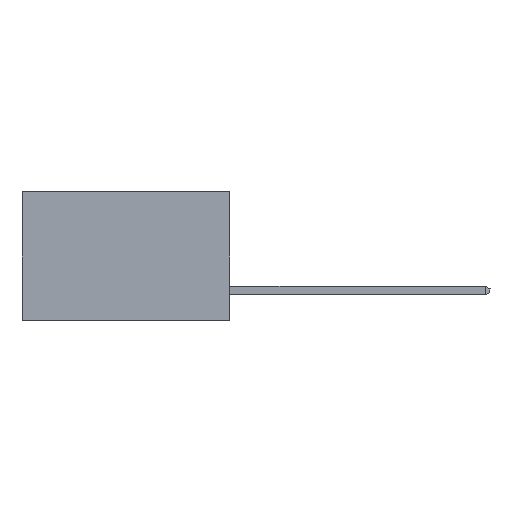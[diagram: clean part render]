
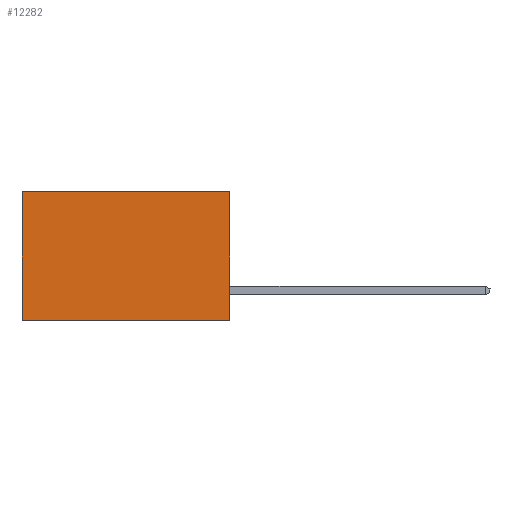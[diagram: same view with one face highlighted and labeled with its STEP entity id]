
A CAD part, left-side view. The second image highlights one B-rep face of the part: STEP entity #12282.
In plain terms, the highlighted planar face has unit normal (-1, 0, 0).
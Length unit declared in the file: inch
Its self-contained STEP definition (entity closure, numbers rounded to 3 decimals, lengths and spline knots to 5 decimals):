
#436 = LINE ( 'NONE', #7657, #5934 ) ;
#659 = ORIENTED_EDGE ( 'NONE', *, *, #10849, .F. ) ;
#1196 = LINE ( 'NONE', #14230, #4941 ) ;
#1981 = ORIENTED_EDGE ( 'NONE', *, *, #10975, .F. ) ;
#3403 = CARTESIAN_POINT ( 'NONE',  ( 0.2615, 0., -0.37 ) ) ;
#3485 = CARTESIAN_POINT ( 'NONE',  ( 0.2615, 0., -0.37 ) ) ;
#4744 = VERTEX_POINT ( 'NONE', #11802 ) ;
#4941 = VECTOR ( 'NONE', #8578, 39.37008 ) ;
#5934 = VECTOR ( 'NONE', #12455, 39.37008 ) ;
#6641 = EDGE_LOOP ( 'NONE', ( #12368, #1981, #659, #8754 ) ) ;
#7217 = EDGE_CURVE ( 'NONE', #10637, #8320, #1196, .T. ) ;
#7335 = CARTESIAN_POINT ( 'NONE',  ( 0.2615, 0.6, 0. ) ) ;
#7657 = CARTESIAN_POINT ( 'NONE',  ( 0.2615, 0., -0.37 ) ) ;
#8320 = VERTEX_POINT ( 'NONE', #14591 ) ;
#8326 = DIRECTION ( 'NONE',  ( 1., 0., 0. ) ) ;
#8578 = DIRECTION ( 'NONE',  ( 0., 0., -1. ) ) ;
#8694 = AXIS2_PLACEMENT_3D ( 'NONE', #3485, #8326, #13577 ) ;
#8754 = ORIENTED_EDGE ( 'NONE', *, *, #12151, .T. ) ;
#9497 = FACE_OUTER_BOUND ( 'NONE', #6641, .T. ) ;
#9571 = DIRECTION ( 'NONE',  ( 0., 0., -1. ) ) ;
#9938 = VECTOR ( 'NONE', #9571, 39.37008 ) ;
#10187 = VECTOR ( 'NONE', #13354, 39.37008 ) ;
#10637 = VERTEX_POINT ( 'NONE', #7335 ) ;
#10849 = EDGE_CURVE ( 'NONE', #4744, #14959, #10902, .T. ) ;
#10902 = LINE ( 'NONE', #3403, #9938 ) ;
#10911 = CARTESIAN_POINT ( 'NONE',  ( 0.2615, 0., 0. ) ) ;
#10975 = EDGE_CURVE ( 'NONE', #14959, #8320, #436, .T. ) ;
#11802 = CARTESIAN_POINT ( 'NONE',  ( 0.2615, 0., 0. ) ) ;
#12092 = LINE ( 'NONE', #10911, #10187 ) ;
#12151 = EDGE_CURVE ( 'NONE', #4744, #10637, #12092, .T. ) ;
#12282 = ADVANCED_FACE ( 'NONE', ( #9497 ), #14281, .F. ) ;
#12368 = ORIENTED_EDGE ( 'NONE', *, *, #7217, .T. ) ;
#12455 = DIRECTION ( 'NONE',  ( 0., 1., 0. ) ) ;
#13354 = DIRECTION ( 'NONE',  ( 0., 1., 0. ) ) ;
#13577 = DIRECTION ( 'NONE',  ( 0., 0., -1. ) ) ;
#13813 = CARTESIAN_POINT ( 'NONE',  ( 0.2615, 0., -0.37 ) ) ;
#14230 = CARTESIAN_POINT ( 'NONE',  ( 0.2615, 0.6, -0.37 ) ) ;
#14281 = PLANE ( 'NONE',  #8694 ) ;
#14591 = CARTESIAN_POINT ( 'NONE',  ( 0.2615, 0.6, -0.37 ) ) ;
#14959 = VERTEX_POINT ( 'NONE', #13813 ) ;
